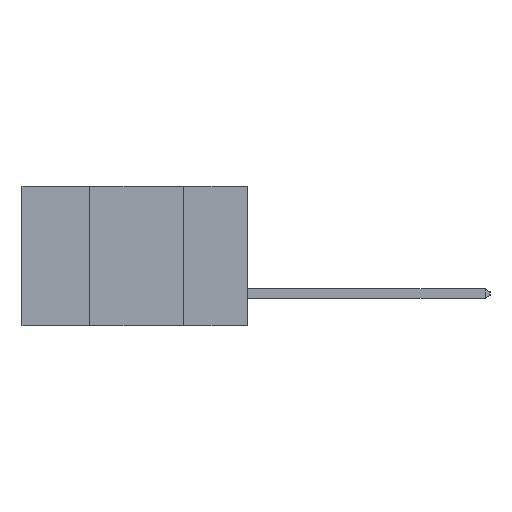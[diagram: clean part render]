
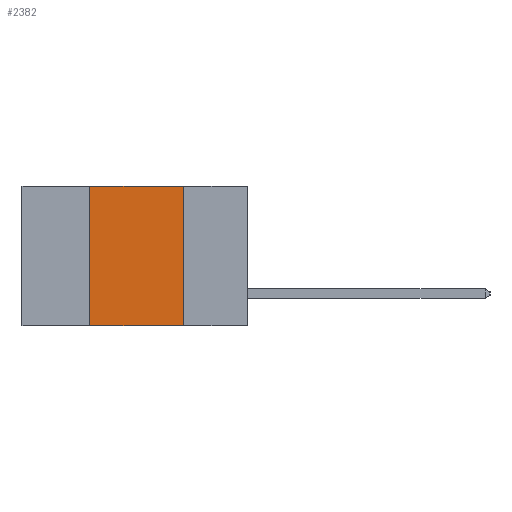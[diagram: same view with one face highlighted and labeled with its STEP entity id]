
A CAD part, left-side view. The second image highlights one B-rep face of the part: STEP entity #2382.
In plain terms, the highlighted planar face has unit normal (-1, 0, 0).
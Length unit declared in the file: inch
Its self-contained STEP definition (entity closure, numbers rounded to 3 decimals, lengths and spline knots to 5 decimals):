
#203 = VERTEX_POINT ( 'NONE', #13294 ) ;
#278 = CARTESIAN_POINT ( 'NONE',  ( 0., 0.17, 0. ) ) ;
#557 = CARTESIAN_POINT ( 'NONE',  ( 0., 0.6, 0. ) ) ;
#877 = DIRECTION ( 'NONE',  ( 0., -1., 0. ) ) ;
#1771 = LINE ( 'NONE', #278, #9837 ) ;
#1835 = LINE ( 'NONE', #5006, #8118 ) ;
#2007 = EDGE_LOOP ( 'NONE', ( #13307, #6340, #10138, #7856 ) ) ;
#2382 = ADVANCED_FACE ( 'NONE', ( #11539 ), #10229, .F. ) ;
#2729 = CARTESIAN_POINT ( 'NONE',  ( 0., 0.17, -0.37 ) ) ;
#2824 = LINE ( 'NONE', #13208, #8438 ) ;
#3409 = CARTESIAN_POINT ( 'NONE',  ( 0., 0.42, -0.37 ) ) ;
#4878 = DIRECTION ( 'NONE',  ( 0., 0., 1. ) ) ;
#5005 = CARTESIAN_POINT ( 'NONE',  ( 0., 0.42, 0. ) ) ;
#5006 = CARTESIAN_POINT ( 'NONE',  ( 0., 0.6, -0.37 ) ) ;
#5301 = VERTEX_POINT ( 'NONE', #5005 ) ;
#6208 = CARTESIAN_POINT ( 'NONE',  ( 0., 0.6, 0. ) ) ;
#6340 = ORIENTED_EDGE ( 'NONE', *, *, #12649, .F. ) ;
#6425 = VERTEX_POINT ( 'NONE', #2729 ) ;
#6436 = EDGE_CURVE ( 'NONE', #6854, #5301, #2824, .T. ) ;
#6506 = EDGE_CURVE ( 'NONE', #6854, #6425, #1835, .T. ) ;
#6626 = DIRECTION ( 'NONE',  ( 0., 0., -1. ) ) ;
#6854 = VERTEX_POINT ( 'NONE', #3409 ) ;
#7856 = ORIENTED_EDGE ( 'NONE', *, *, #6506, .T. ) ;
#8118 = VECTOR ( 'NONE', #11250, 39.37008 ) ;
#8438 = VECTOR ( 'NONE', #4878, 39.37008 ) ;
#9040 = AXIS2_PLACEMENT_3D ( 'NONE', #557, #11311, #11367 ) ;
#9441 = VECTOR ( 'NONE', #877, 39.37008 ) ;
#9837 = VECTOR ( 'NONE', #6626, 39.37008 ) ;
#10138 = ORIENTED_EDGE ( 'NONE', *, *, #6436, .F. ) ;
#10229 = PLANE ( 'NONE',  #9040 ) ;
#10674 = EDGE_CURVE ( 'NONE', #203, #6425, #1771, .T. ) ;
#11250 = DIRECTION ( 'NONE',  ( 0., -1., 0. ) ) ;
#11311 = DIRECTION ( 'NONE',  ( 1., 0., 0. ) ) ;
#11367 = DIRECTION ( 'NONE',  ( 0., 0., -1. ) ) ;
#11539 = FACE_OUTER_BOUND ( 'NONE', #2007, .T. ) ;
#11554 = LINE ( 'NONE', #6208, #9441 ) ;
#12649 = EDGE_CURVE ( 'NONE', #5301, #203, #11554, .T. ) ;
#13208 = CARTESIAN_POINT ( 'NONE',  ( 0., 0.42, 0. ) ) ;
#13294 = CARTESIAN_POINT ( 'NONE',  ( 0., 0.17, 0. ) ) ;
#13307 = ORIENTED_EDGE ( 'NONE', *, *, #10674, .F. ) ;
